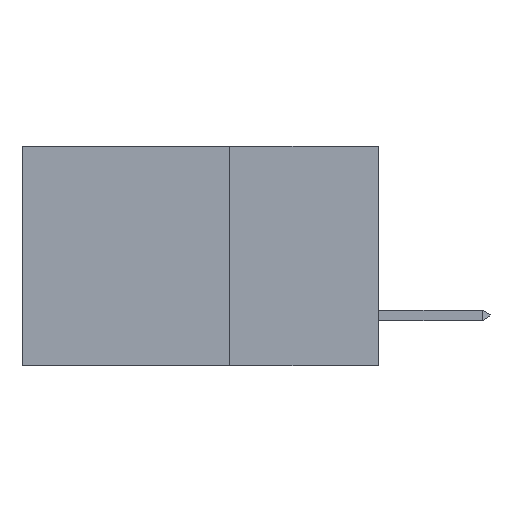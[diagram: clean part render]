
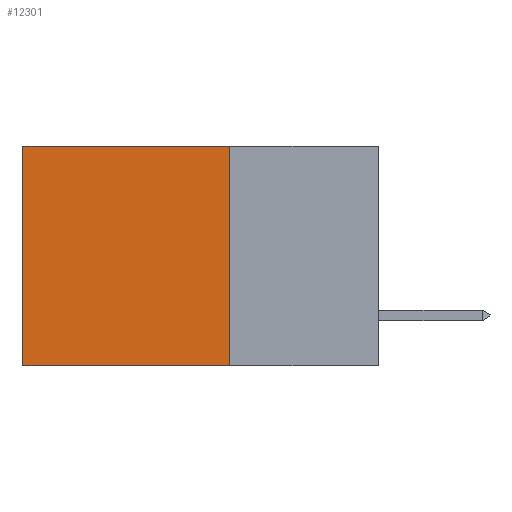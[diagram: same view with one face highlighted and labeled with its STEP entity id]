
A CAD part, left-side view. The second image highlights one B-rep face of the part: STEP entity #12301.
In plain terms, the highlighted planar face has unit normal (-1, 0, 0).
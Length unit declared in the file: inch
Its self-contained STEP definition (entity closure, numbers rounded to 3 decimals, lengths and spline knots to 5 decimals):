
#330 = CARTESIAN_POINT ( 'NONE',  ( 0.298, 0.25, 0. ) ) ;
#530 = CARTESIAN_POINT ( 'NONE',  ( 0.298, 0.25, -0.37 ) ) ;
#537 = VERTEX_POINT ( 'NONE', #3507 ) ;
#1142 = EDGE_LOOP ( 'NONE', ( #16695, #6881, #3229, #16555 ) ) ;
#2075 = LINE ( 'NONE', #12134, #10441 ) ;
#2540 = EDGE_CURVE ( 'NONE', #17145, #10483, #2075, .T. ) ;
#3023 = VERTEX_POINT ( 'NONE', #17764 ) ;
#3229 = ORIENTED_EDGE ( 'NONE', *, *, #12118, .F. ) ;
#3259 = DIRECTION ( 'NONE',  ( 1., 0., 0. ) ) ;
#3287 = VECTOR ( 'NONE', #5506, 39.37008 ) ;
#3507 = CARTESIAN_POINT ( 'NONE',  ( 0.298, 0.6, -0.37 ) ) ;
#4175 = DIRECTION ( 'NONE',  ( 0., 0., -1. ) ) ;
#4896 = AXIS2_PLACEMENT_3D ( 'NONE', #10219, #3259, #7356 ) ;
#5178 = DIRECTION ( 'NONE',  ( 0., 1., 0. ) ) ;
#5506 = DIRECTION ( 'NONE',  ( 0., 0., -1. ) ) ;
#6649 = CARTESIAN_POINT ( 'NONE',  ( 0.298, 0.25, 0. ) ) ;
#6881 = ORIENTED_EDGE ( 'NONE', *, *, #10463, .F. ) ;
#7356 = DIRECTION ( 'NONE',  ( 0., 0., -1. ) ) ;
#10219 = CARTESIAN_POINT ( 'NONE',  ( 0.298, 0.25, 0. ) ) ;
#10441 = VECTOR ( 'NONE', #5178, 39.37008 ) ;
#10463 = EDGE_CURVE ( 'NONE', #3023, #537, #10726, .T. ) ;
#10483 = VERTEX_POINT ( 'NONE', #11135 ) ;
#10719 = EDGE_CURVE ( 'NONE', #10483, #537, #11143, .T. ) ;
#10726 = LINE ( 'NONE', #530, #12662 ) ;
#11135 = CARTESIAN_POINT ( 'NONE',  ( 0.298, 0.6, 0. ) ) ;
#11143 = LINE ( 'NONE', #12390, #15274 ) ;
#12118 = EDGE_CURVE ( 'NONE', #17145, #3023, #14372, .T. ) ;
#12134 = CARTESIAN_POINT ( 'NONE',  ( 0.298, 0.25, 0. ) ) ;
#12301 = ADVANCED_FACE ( 'NONE', ( #16633 ), #15602, .F. ) ;
#12390 = CARTESIAN_POINT ( 'NONE',  ( 0.298, 0.6, 0. ) ) ;
#12662 = VECTOR ( 'NONE', #12840, 39.37008 ) ;
#12840 = DIRECTION ( 'NONE',  ( 0., 1., 0. ) ) ;
#14372 = LINE ( 'NONE', #6649, #3287 ) ;
#15274 = VECTOR ( 'NONE', #4175, 39.37008 ) ;
#15602 = PLANE ( 'NONE',  #4896 ) ;
#16555 = ORIENTED_EDGE ( 'NONE', *, *, #2540, .T. ) ;
#16633 = FACE_OUTER_BOUND ( 'NONE', #1142, .T. ) ;
#16695 = ORIENTED_EDGE ( 'NONE', *, *, #10719, .T. ) ;
#17145 = VERTEX_POINT ( 'NONE', #330 ) ;
#17764 = CARTESIAN_POINT ( 'NONE',  ( 0.298, 0.25, -0.37 ) ) ;
